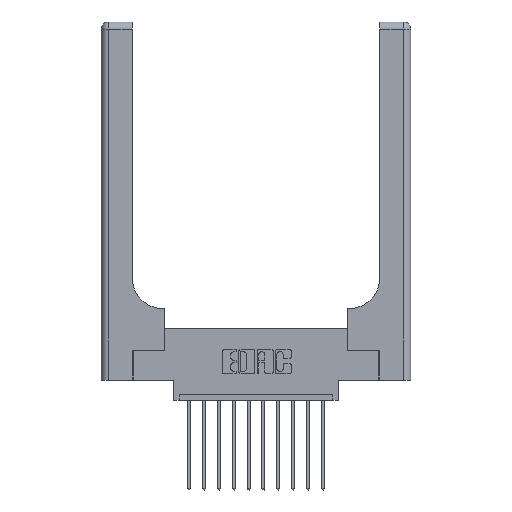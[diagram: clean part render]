
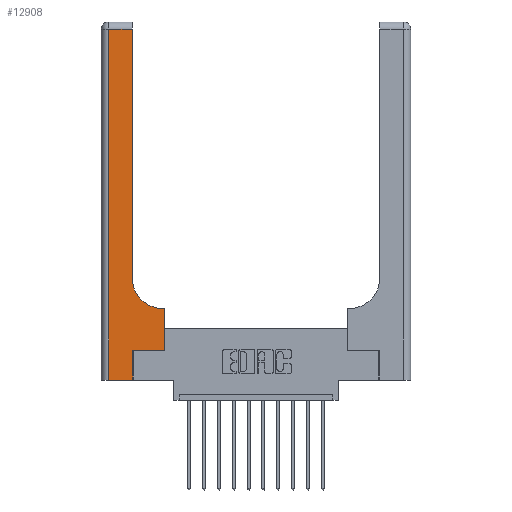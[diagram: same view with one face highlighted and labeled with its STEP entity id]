
A CAD part, top view. The second image highlights one B-rep face of the part: STEP entity #12908.
In plain terms, the highlighted planar face has unit normal (0, 0, 1).
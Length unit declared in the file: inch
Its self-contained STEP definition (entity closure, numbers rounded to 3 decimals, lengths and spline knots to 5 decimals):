
#34 = CARTESIAN_POINT ( 'NONE',  ( 0.26, 3., 0.37 ) ) ;
#372 = LINE ( 'NONE', #4249, #4310 ) ;
#433 = VECTOR ( 'NONE', #2836, 39.37008 ) ;
#476 = DIRECTION ( 'NONE',  ( -1., 0., 0. ) ) ;
#517 = FACE_OUTER_BOUND ( 'NONE', #15127, .T. ) ;
#825 = ORIENTED_EDGE ( 'NONE', *, *, #5344, .T. ) ;
#1136 = VERTEX_POINT ( 'NONE', #14571 ) ;
#1199 = DIRECTION ( 'NONE',  ( 0., 1., 0. ) ) ;
#1327 = VECTOR ( 'NONE', #1199, 39.37008 ) ;
#1524 = CARTESIAN_POINT ( 'NONE',  ( 0.51, 0.6, 0.37 ) ) ;
#1668 = VERTEX_POINT ( 'NONE', #3436 ) ;
#1762 = VERTEX_POINT ( 'NONE', #14699 ) ;
#1823 = CARTESIAN_POINT ( 'NONE',  ( 0., 3., 0.37 ) ) ;
#1910 = EDGE_CURVE ( 'NONE', #10400, #14338, #4094, .T. ) ;
#2097 = ORIENTED_EDGE ( 'NONE', *, *, #1910, .T. ) ;
#2132 = VECTOR ( 'NONE', #14130, 39.37008 ) ;
#2595 = EDGE_CURVE ( 'NONE', #12400, #1136, #6631, .T. ) ;
#2722 = VERTEX_POINT ( 'NONE', #15032 ) ;
#2829 = VERTEX_POINT ( 'NONE', #8129 ) ;
#2836 = DIRECTION ( 'NONE',  ( 1., 0., 0. ) ) ;
#3096 = VECTOR ( 'NONE', #13474, 39.37008 ) ;
#3386 = VECTOR ( 'NONE', #4344, 39.37008 ) ;
#3436 = CARTESIAN_POINT ( 'NONE',  ( 0.265, 0.25, 0.37 ) ) ;
#3837 = CARTESIAN_POINT ( 'NONE',  ( 0., 2.94, 0.37 ) ) ;
#4094 = LINE ( 'NONE', #3837, #2132 ) ;
#4179 = EDGE_CURVE ( 'NONE', #1136, #10400, #9535, .T. ) ;
#4249 = CARTESIAN_POINT ( 'NONE',  ( 0.06, 3., 0.37 ) ) ;
#4274 = CARTESIAN_POINT ( 'NONE',  ( 0.26, 0.6, 0.37 ) ) ;
#4310 = VECTOR ( 'NONE', #11657, 39.37008 ) ;
#4344 = DIRECTION ( 'NONE',  ( 0., 1., 0. ) ) ;
#4425 = EDGE_CURVE ( 'NONE', #14338, #1762, #372, .T. ) ;
#5326 = LINE ( 'NONE', #14118, #10738 ) ;
#5341 = CARTESIAN_POINT ( 'NONE',  ( 0.528, 0.25, 0.37 ) ) ;
#5344 = EDGE_CURVE ( 'NONE', #1668, #2722, #15435, .T. ) ;
#5514 = LINE ( 'NONE', #4274, #15757 ) ;
#5745 = ORIENTED_EDGE ( 'NONE', *, *, #4425, .T. ) ;
#6631 = CIRCLE ( 'NONE', #14255, 0.25 ) ;
#6991 = VERTEX_POINT ( 'NONE', #11205 ) ;
#7763 = EDGE_CURVE ( 'NONE', #1762, #2829, #14114, .T. ) ;
#8129 = CARTESIAN_POINT ( 'NONE',  ( 0.265, 0., 0.37 ) ) ;
#8929 = CARTESIAN_POINT ( 'NONE',  ( 0., 0., 0.37 ) ) ;
#9535 = LINE ( 'NONE', #34, #1327 ) ;
#9555 = CARTESIAN_POINT ( 'NONE',  ( 0.06, 2.94, 0.37 ) ) ;
#9709 = CARTESIAN_POINT ( 'NONE',  ( 0.51, 0.85, 0.37 ) ) ;
#10320 = DIRECTION ( 'NONE',  ( 0., 0., -1. ) ) ;
#10379 = ORIENTED_EDGE ( 'NONE', *, *, #7763, .T. ) ;
#10400 = VERTEX_POINT ( 'NONE', #15407 ) ;
#10738 = VECTOR ( 'NONE', #12876, 39.37008 ) ;
#11131 = EDGE_CURVE ( 'NONE', #2722, #6991, #14136, .T. ) ;
#11205 = CARTESIAN_POINT ( 'NONE',  ( 0.528, 0.6, 0.37 ) ) ;
#11383 = EDGE_CURVE ( 'NONE', #2829, #1668, #5326, .T. ) ;
#11657 = DIRECTION ( 'NONE',  ( 0., -1., 0. ) ) ;
#12080 = ORIENTED_EDGE ( 'NONE', *, *, #11131, .T. ) ;
#12400 = VERTEX_POINT ( 'NONE', #1524 ) ;
#12403 = CARTESIAN_POINT ( 'NONE',  ( 0.265, 0.25, 0.37 ) ) ;
#12876 = DIRECTION ( 'NONE',  ( 0., 1., 0. ) ) ;
#12908 = ADVANCED_FACE ( 'NONE', ( #517 ), #13025, .F. ) ;
#13025 = PLANE ( 'NONE',  #14192 ) ;
#13106 = DIRECTION ( 'NONE',  ( -1., 0., 0. ) ) ;
#13322 = DIRECTION ( 'NONE',  ( 0., 0., -1. ) ) ;
#13469 = ORIENTED_EDGE ( 'NONE', *, *, #4179, .T. ) ;
#13474 = DIRECTION ( 'NONE',  ( 1., 0., 0. ) ) ;
#13645 = DIRECTION ( 'NONE',  ( 1., 0., 0. ) ) ;
#14114 = LINE ( 'NONE', #8929, #433 ) ;
#14118 = CARTESIAN_POINT ( 'NONE',  ( 0.265, 0., 0.37 ) ) ;
#14130 = DIRECTION ( 'NONE',  ( -1., 0., 0. ) ) ;
#14136 = LINE ( 'NONE', #5341, #3386 ) ;
#14192 = AXIS2_PLACEMENT_3D ( 'NONE', #1823, #10320, #13106 ) ;
#14255 = AXIS2_PLACEMENT_3D ( 'NONE', #9709, #13322, #13645 ) ;
#14338 = VERTEX_POINT ( 'NONE', #9555 ) ;
#14571 = CARTESIAN_POINT ( 'NONE',  ( 0.26, 0.85, 0.37 ) ) ;
#14574 = EDGE_CURVE ( 'NONE', #6991, #12400, #5514, .T. ) ;
#14699 = CARTESIAN_POINT ( 'NONE',  ( 0.06, 0., 0.37 ) ) ;
#14963 = ORIENTED_EDGE ( 'NONE', *, *, #14574, .T. ) ;
#15032 = CARTESIAN_POINT ( 'NONE',  ( 0.528, 0.25, 0.37 ) ) ;
#15127 = EDGE_LOOP ( 'NONE', ( #13469, #2097, #5745, #10379, #15684, #825, #12080, #14963, #15219 ) ) ;
#15219 = ORIENTED_EDGE ( 'NONE', *, *, #2595, .T. ) ;
#15407 = CARTESIAN_POINT ( 'NONE',  ( 0.26, 2.94, 0.37 ) ) ;
#15435 = LINE ( 'NONE', #12403, #3096 ) ;
#15684 = ORIENTED_EDGE ( 'NONE', *, *, #11383, .T. ) ;
#15757 = VECTOR ( 'NONE', #476, 39.37008 ) ;
